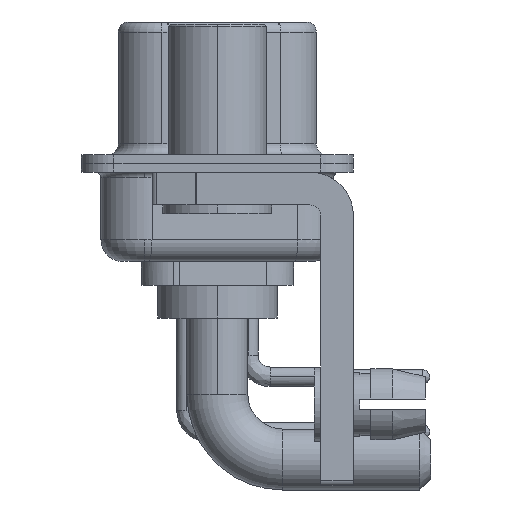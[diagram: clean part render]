
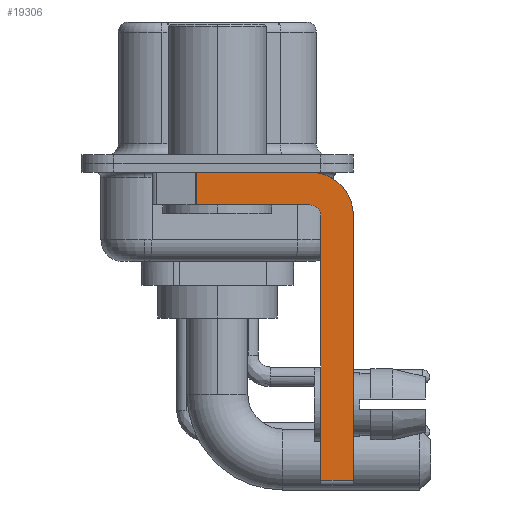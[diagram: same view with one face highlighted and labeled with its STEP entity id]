
A CAD part, left-side view. The second image highlights one B-rep face of the part: STEP entity #19306.
In plain terms, the highlighted planar face has unit normal (-1, 0, 0).
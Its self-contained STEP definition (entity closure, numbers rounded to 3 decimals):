
#38 = EDGE_CURVE ( 'NONE', #13076, #30467, #31577, .T. ) ;
#666 = EDGE_LOOP ( 'NONE', ( #28820, #18701, #1980, #2139, #28436, #24968, #17494, #5932 ) ) ;
#724 = VERTEX_POINT ( 'NONE', #11265 ) ;
#1239 = FACE_OUTER_BOUND ( 'NONE', #666, .T. ) ;
#1812 = VECTOR ( 'NONE', #14682, 1000. ) ;
#1980 = ORIENTED_EDGE ( 'NONE', *, *, #30591, .F. ) ;
#2139 = ORIENTED_EDGE ( 'NONE', *, *, #30821, .F. ) ;
#2354 = CIRCLE ( 'NONE', #20508, 0.5 ) ;
#3480 = EDGE_CURVE ( 'NONE', #23387, #724, #29416, .T. ) ;
#3633 = CARTESIAN_POINT ( 'NONE',  ( -2.9, -4.25, -1.9 ) ) ;
#3967 = DIRECTION ( 'NONE',  ( -1., 0., 0. ) ) ;
#4285 = EDGE_CURVE ( 'NONE', #23387, #23803, #29422, .T. ) ;
#5932 = ORIENTED_EDGE ( 'NONE', *, *, #38, .F. ) ;
#6165 = EDGE_CURVE ( 'NONE', #15417, #13076, #23078, .T. ) ;
#7515 = VECTOR ( 'NONE', #22798, 1000. ) ;
#7820 = CARTESIAN_POINT ( 'NONE',  ( -2.9, 0.978, -0.4 ) ) ;
#8136 = DIRECTION ( 'NONE',  ( 0., -1., 0. ) ) ;
#8710 = DIRECTION ( 'NONE',  ( 1., 0., 0. ) ) ;
#8880 = CARTESIAN_POINT ( 'NONE',  ( -2.9, -4.25, -2.4 ) ) ;
#9291 = DIRECTION ( 'NONE',  ( 0., 0., -1. ) ) ;
#9490 = CARTESIAN_POINT ( 'NONE',  ( -2.9, -4.25, -14.55 ) ) ;
#9810 = DIRECTION ( 'NONE',  ( 0., 0., 1. ) ) ;
#10303 = CARTESIAN_POINT ( 'NONE',  ( -2.9, -6.25, -2.4 ) ) ;
#11151 = DIRECTION ( 'NONE',  ( 0., 0., -1. ) ) ;
#11265 = CARTESIAN_POINT ( 'NONE',  ( -2.9, -6.25, -14.55 ) ) ;
#11419 = DIRECTION ( 'NONE',  ( 0., 0., 1. ) ) ;
#11857 = VERTEX_POINT ( 'NONE', #29739 ) ;
#12136 = EDGE_CURVE ( 'NONE', #15417, #11857, #21658, .T. ) ;
#12339 = CARTESIAN_POINT ( 'NONE',  ( -2.9, -4.25, -2.4 ) ) ;
#12908 = LINE ( 'NONE', #10303, #18303 ) ;
#13076 = VERTEX_POINT ( 'NONE', #27483 ) ;
#14682 = DIRECTION ( 'NONE',  ( 0., -1., 0. ) ) ;
#15358 = DIRECTION ( 'NONE',  ( 0., 0., -1. ) ) ;
#15417 = VERTEX_POINT ( 'NONE', #7820 ) ;
#15978 = LINE ( 'NONE', #3633, #7515 ) ;
#16027 = VECTOR ( 'NONE', #8136, 1000. ) ;
#16752 = DIRECTION ( 'NONE',  ( 0., 0., -1. ) ) ;
#17228 = DIRECTION ( 'NONE',  ( 1., 0., 0. ) ) ;
#17494 = ORIENTED_EDGE ( 'NONE', *, *, #28199, .F. ) ;
#18303 = VECTOR ( 'NONE', #15358, 1000. ) ;
#18701 = ORIENTED_EDGE ( 'NONE', *, *, #12136, .T. ) ;
#19306 = ADVANCED_FACE ( 'NONE', ( #1239 ), #31077, .F. ) ;
#19981 = VECTOR ( 'NONE', #9291, 1000. ) ;
#20508 = AXIS2_PLACEMENT_3D ( 'NONE', #26022, #3967, #11419 ) ;
#21418 = AXIS2_PLACEMENT_3D ( 'NONE', #8880, #8710, #11151 ) ;
#21658 = LINE ( 'NONE', #31011, #19981 ) ;
#22798 = DIRECTION ( 'NONE',  ( 0., 1., 0. ) ) ;
#22916 = CARTESIAN_POINT ( 'NONE',  ( -2.9, 3., -0.4 ) ) ;
#23078 = LINE ( 'NONE', #22916, #16027 ) ;
#23387 = VERTEX_POINT ( 'NONE', #25968 ) ;
#23629 = VECTOR ( 'NONE', #9810, 1000. ) ;
#23803 = VERTEX_POINT ( 'NONE', #28247 ) ;
#24968 = ORIENTED_EDGE ( 'NONE', *, *, #3480, .T. ) ;
#25968 = CARTESIAN_POINT ( 'NONE',  ( -2.9, -4.75, -14.55 ) ) ;
#26022 = CARTESIAN_POINT ( 'NONE',  ( -2.9, -4.25, -2.4 ) ) ;
#26844 = CARTESIAN_POINT ( 'NONE',  ( -2.9, -4.75, -14.8 ) ) ;
#26852 = CARTESIAN_POINT ( 'NONE',  ( -2.9, -6.25, -2.4 ) ) ;
#27483 = CARTESIAN_POINT ( 'NONE',  ( -2.9, -4.25, -0.4 ) ) ;
#28199 = EDGE_CURVE ( 'NONE', #30467, #724, #12908, .T. ) ;
#28247 = CARTESIAN_POINT ( 'NONE',  ( -2.9, -4.75, -2.4 ) ) ;
#28436 = ORIENTED_EDGE ( 'NONE', *, *, #4285, .F. ) ;
#28820 = ORIENTED_EDGE ( 'NONE', *, *, #6165, .F. ) ;
#29416 = LINE ( 'NONE', #9490, #1812 ) ;
#29422 = LINE ( 'NONE', #26844, #23629 ) ;
#29739 = CARTESIAN_POINT ( 'NONE',  ( -2.9, 0.978, -1.9 ) ) ;
#30130 = CARTESIAN_POINT ( 'NONE',  ( -2.9, -4.25, -1.9 ) ) ;
#30467 = VERTEX_POINT ( 'NONE', #26852 ) ;
#30591 = EDGE_CURVE ( 'NONE', #31474, #11857, #15978, .T. ) ;
#30821 = EDGE_CURVE ( 'NONE', #23803, #31474, #2354, .T. ) ;
#31011 = CARTESIAN_POINT ( 'NONE',  ( -2.9, 0.978, -1.9 ) ) ;
#31067 = AXIS2_PLACEMENT_3D ( 'NONE', #12339, #17228, #16752 ) ;
#31077 = PLANE ( 'NONE',  #21418 ) ;
#31474 = VERTEX_POINT ( 'NONE', #30130 ) ;
#31577 = CIRCLE ( 'NONE', #31067, 2. ) ;
